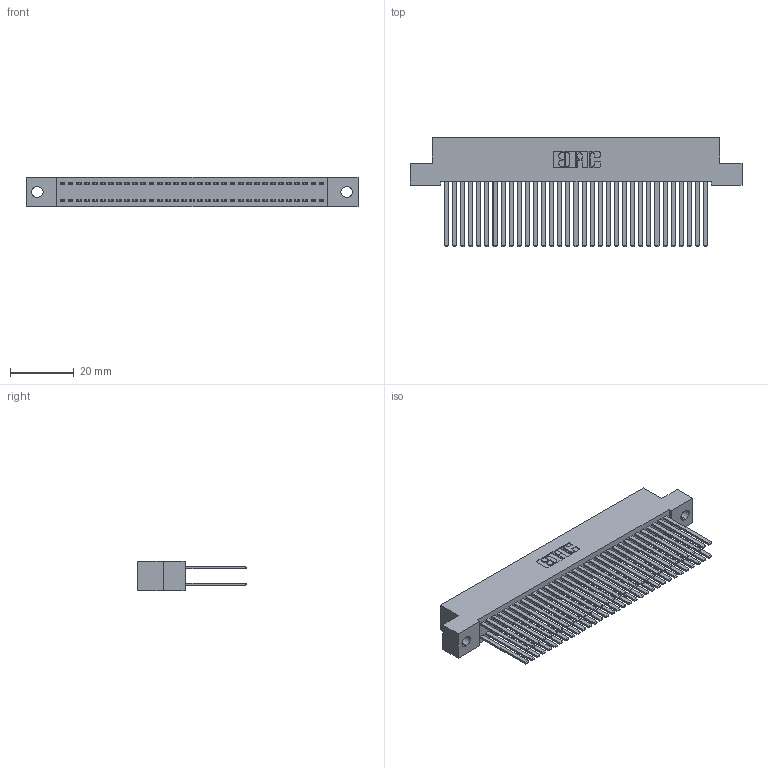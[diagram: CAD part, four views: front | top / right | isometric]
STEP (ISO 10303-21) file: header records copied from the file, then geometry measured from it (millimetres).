
FILE_DESCRIPTION (( 'STEP AP203' ), '1' );
FILE_NAME ('342-066-544-202.STEP', '2018-08-13T08:08:37', ( '' ), ( '' ), 'SwSTEP 2.0', 'SolidWorks 2016', '' );
FILE_SCHEMA (( 'CONFIG_CONTROL_DESIGN' ));
Length unit declared in the file: inch
Products named in the file (3): 342 Part_.128 Slot; 345-292-001_345-293-144; 342-066-544-202
Assembly tree (67 placements, depth 2):
  342-066-544-202
    342 Part_.128 Slot
    345-292-001_345-293-144  x66
Bounding box: 104.14 x 34.3 x 9.4 mm (x, y, z)
Volume: 10187.4 mm3; surface area: 18682.5 mm2
Topology: 67 solids, 67 shells, 3150 faces, 9353 edges, 6146 vertices
Faces by surface type: plane 2182, cylinder 968
Entity records: 22213 total; most frequent: CARTESIAN_POINT 3690, ORIENTED_EDGE 3626, DIRECTION 3165, EDGE_CURVE 1813, LINE 1689, VECTOR 1689, VERTEX_POINT 1206, AXIS2_PLACEMENT_3D 738
